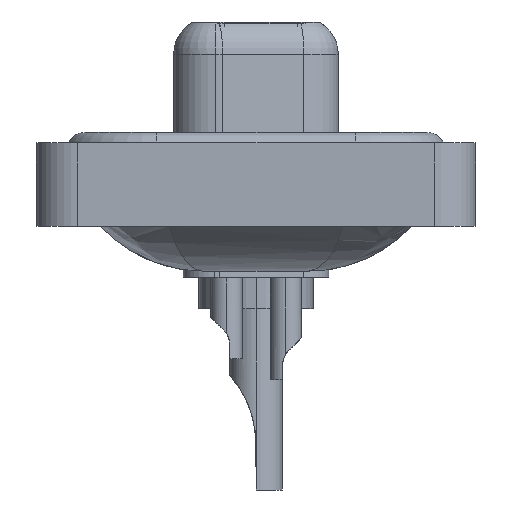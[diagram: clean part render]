
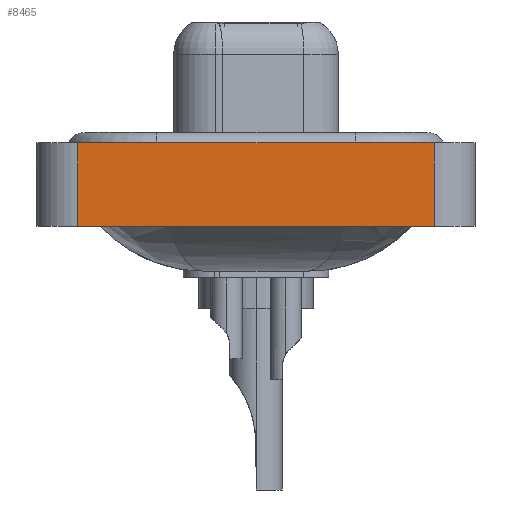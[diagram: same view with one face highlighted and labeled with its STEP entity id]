
A CAD part, left-side view. The second image highlights one B-rep face of the part: STEP entity #8465.
In plain terms, the highlighted planar face has unit normal (-1, 0, 0).
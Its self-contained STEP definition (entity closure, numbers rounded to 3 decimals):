
#495 = VERTEX_POINT ( 'NONE', #2595 ) ;
#2595 = CARTESIAN_POINT ( 'NONE',  ( -7.35, 8.55, -3.6 ) ) ;
#2788 = LINE ( 'NONE', #14836, #8844 ) ;
#3322 = ORIENTED_EDGE ( 'NONE', *, *, #13343, .F. ) ;
#3323 = VECTOR ( 'NONE', #20600, 1000. ) ;
#5389 = VECTOR ( 'NONE', #13246, 1000. ) ;
#5744 = EDGE_CURVE ( 'NONE', #19961, #24096, #25395, .T. ) ;
#8465 = ADVANCED_FACE ( 'NONE', ( #15976 ), #13977, .T. ) ;
#8844 = VECTOR ( 'NONE', #18968, 1000. ) ;
#9403 = CARTESIAN_POINT ( 'NONE',  ( -7.35, -8.55, 0.4 ) ) ;
#10675 = EDGE_CURVE ( 'NONE', #14411, #24096, #26201, .T. ) ;
#10845 = CARTESIAN_POINT ( 'NONE',  ( -7.35, -8.55, -3.6 ) ) ;
#10895 = EDGE_CURVE ( 'NONE', #495, #19961, #2788, .T. ) ;
#12588 = ORIENTED_EDGE ( 'NONE', *, *, #10675, .F. ) ;
#13246 = DIRECTION ( 'NONE',  ( 0., 0., 1. ) ) ;
#13343 = EDGE_CURVE ( 'NONE', #495, #14411, #22877, .T. ) ;
#13795 = ORIENTED_EDGE ( 'NONE', *, *, #5744, .T. ) ;
#13930 = VECTOR ( 'NONE', #23935, 1000. ) ;
#13977 = PLANE ( 'NONE',  #21490 ) ;
#14411 = VERTEX_POINT ( 'NONE', #20286 ) ;
#14836 = CARTESIAN_POINT ( 'NONE',  ( -7.35, -8.55, -3.6 ) ) ;
#15631 = ORIENTED_EDGE ( 'NONE', *, *, #10895, .T. ) ;
#15976 = FACE_OUTER_BOUND ( 'NONE', #17883, .T. ) ;
#16469 = CARTESIAN_POINT ( 'NONE',  ( -7.35, 8.55, -3.6 ) ) ;
#17722 = CARTESIAN_POINT ( 'NONE',  ( -7.35, -8.55, -3.6 ) ) ;
#17883 = EDGE_LOOP ( 'NONE', ( #13795, #12588, #3322, #15631 ) ) ;
#18968 = DIRECTION ( 'NONE',  ( 0., -1., 0. ) ) ;
#19840 = DIRECTION ( 'NONE',  ( -1., 0., 0. ) ) ;
#19917 = CARTESIAN_POINT ( 'NONE',  ( -7.35, -8.55, 0.4 ) ) ;
#19961 = VERTEX_POINT ( 'NONE', #10845 ) ;
#20286 = CARTESIAN_POINT ( 'NONE',  ( -7.35, 8.55, 0.4 ) ) ;
#20600 = DIRECTION ( 'NONE',  ( 0., 0., 1. ) ) ;
#21490 = AXIS2_PLACEMENT_3D ( 'NONE', #17722, #19840, #22243 ) ;
#22243 = DIRECTION ( 'NONE',  ( 0., 0., 1. ) ) ;
#22877 = LINE ( 'NONE', #16469, #3323 ) ;
#23658 = CARTESIAN_POINT ( 'NONE',  ( -7.35, -8.55, -3.6 ) ) ;
#23935 = DIRECTION ( 'NONE',  ( 0., -1., 0. ) ) ;
#24096 = VERTEX_POINT ( 'NONE', #9403 ) ;
#25395 = LINE ( 'NONE', #23658, #5389 ) ;
#26201 = LINE ( 'NONE', #19917, #13930 ) ;
